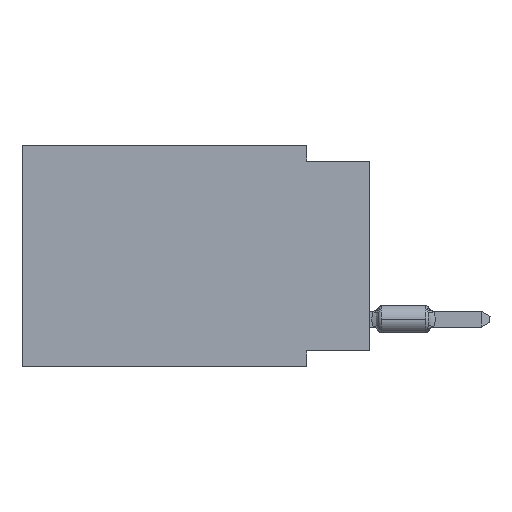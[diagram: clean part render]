
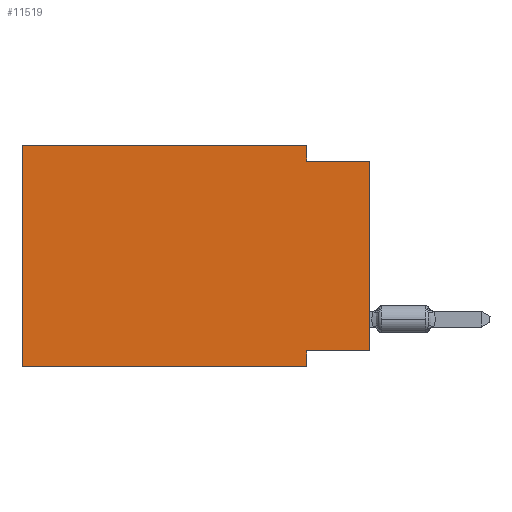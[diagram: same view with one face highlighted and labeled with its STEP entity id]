
A CAD part, left-side view. The second image highlights one B-rep face of the part: STEP entity #11519.
In plain terms, the highlighted planar face has unit normal (-1, 0, 0).
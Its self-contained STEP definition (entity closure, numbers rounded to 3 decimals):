
#225 = EDGE_CURVE ( 'NONE', #2638, #29900, #37555, .T. ) ;
#253 = CARTESIAN_POINT ( 'NONE',  ( 0., 0., -8.255 ) ) ;
#2038 = VECTOR ( 'NONE', #21375, 1000. ) ;
#2461 = CARTESIAN_POINT ( 'NONE',  ( 0., 13.97, -8.89 ) ) ;
#2638 = VERTEX_POINT ( 'NONE', #18817 ) ;
#3577 = DIRECTION ( 'NONE',  ( 1., 0., 0. ) ) ;
#8755 = EDGE_CURVE ( 'NONE', #37932, #35899, #27618, .T. ) ;
#8893 = FACE_OUTER_BOUND ( 'NONE', #53935, .T. ) ;
#9182 = CARTESIAN_POINT ( 'NONE',  ( 0., 2.54, 0. ) ) ;
#10753 = CARTESIAN_POINT ( 'NONE',  ( 0., 2.54, -8.89 ) ) ;
#11464 = VERTEX_POINT ( 'NONE', #9182 ) ;
#11519 = ADVANCED_FACE ( 'NONE', ( #8893 ), #27008, .F. ) ;
#12480 = EDGE_CURVE ( 'NONE', #11464, #40241, #20496, .T. ) ;
#13843 = EDGE_CURVE ( 'NONE', #37932, #29900, #56227, .T. ) ;
#18072 = EDGE_CURVE ( 'NONE', #40241, #25792, #42364, .T. ) ;
#18817 = CARTESIAN_POINT ( 'NONE',  ( 0., 2.54, -8.255 ) ) ;
#18833 = CARTESIAN_POINT ( 'NONE',  ( 0., 2.54, -8.89 ) ) ;
#19452 = CARTESIAN_POINT ( 'NONE',  ( 0., 0., -8.255 ) ) ;
#19778 = CARTESIAN_POINT ( 'NONE',  ( 0., 0., -0.635 ) ) ;
#20298 = VECTOR ( 'NONE', #28694, 1000. ) ;
#20496 = LINE ( 'NONE', #38919, #2038 ) ;
#21157 = VECTOR ( 'NONE', #37764, 1000. ) ;
#21375 = DIRECTION ( 'NONE',  ( 0., 0., -1. ) ) ;
#23720 = AXIS2_PLACEMENT_3D ( 'NONE', #45130, #3577, #57916 ) ;
#25696 = EDGE_CURVE ( 'NONE', #30554, #2638, #42333, .T. ) ;
#25792 = VERTEX_POINT ( 'NONE', #38165 ) ;
#27008 = PLANE ( 'NONE',  #23720 ) ;
#27618 = LINE ( 'NONE', #37426, #53751 ) ;
#28192 = CARTESIAN_POINT ( 'NONE',  ( 0., 13.97, -8.89 ) ) ;
#28514 = LINE ( 'NONE', #51082, #40633 ) ;
#28694 = DIRECTION ( 'NONE',  ( 0., -1., 0. ) ) ;
#29501 = ORIENTED_EDGE ( 'NONE', *, *, #13843, .T. ) ;
#29900 = VERTEX_POINT ( 'NONE', #10753 ) ;
#30554 = VERTEX_POINT ( 'NONE', #253 ) ;
#32705 = CARTESIAN_POINT ( 'NONE',  ( 0., 0., 0. ) ) ;
#33059 = ORIENTED_EDGE ( 'NONE', *, *, #225, .F. ) ;
#33411 = ORIENTED_EDGE ( 'NONE', *, *, #8755, .F. ) ;
#35899 = VERTEX_POINT ( 'NONE', #39149 ) ;
#36910 = VECTOR ( 'NONE', #37587, 1000. ) ;
#37426 = CARTESIAN_POINT ( 'NONE',  ( 0., 13.97, 0. ) ) ;
#37555 = LINE ( 'NONE', #18833, #45721 ) ;
#37587 = DIRECTION ( 'NONE',  ( 0., 1., 0. ) ) ;
#37764 = DIRECTION ( 'NONE',  ( 0., 0., 1. ) ) ;
#37772 = CARTESIAN_POINT ( 'NONE',  ( 0., 2.54, -0.635 ) ) ;
#37932 = VERTEX_POINT ( 'NONE', #28192 ) ;
#38165 = CARTESIAN_POINT ( 'NONE',  ( 0., 0., -0.635 ) ) ;
#38228 = ORIENTED_EDGE ( 'NONE', *, *, #18072, .F. ) ;
#38919 = CARTESIAN_POINT ( 'NONE',  ( 0., 2.54, 0. ) ) ;
#38969 = EDGE_CURVE ( 'NONE', #30554, #25792, #41631, .T. ) ;
#39149 = CARTESIAN_POINT ( 'NONE',  ( 0., 13.97, 0. ) ) ;
#40241 = VERTEX_POINT ( 'NONE', #37772 ) ;
#40633 = VECTOR ( 'NONE', #52232, 1000. ) ;
#41631 = LINE ( 'NONE', #32705, #21157 ) ;
#42333 = LINE ( 'NONE', #19452, #36910 ) ;
#42364 = LINE ( 'NONE', #19778, #20298 ) ;
#45130 = CARTESIAN_POINT ( 'NONE',  ( 0., 13.97, 0. ) ) ;
#45721 = VECTOR ( 'NONE', #55662, 1000. ) ;
#47053 = VECTOR ( 'NONE', #51176, 1000. ) ;
#49844 = ORIENTED_EDGE ( 'NONE', *, *, #38969, .T. ) ;
#51082 = CARTESIAN_POINT ( 'NONE',  ( 0., 13.97, 0. ) ) ;
#51176 = DIRECTION ( 'NONE',  ( 0., -1., 0. ) ) ;
#52232 = DIRECTION ( 'NONE',  ( 0., -1., 0. ) ) ;
#53751 = VECTOR ( 'NONE', #55534, 1000. ) ;
#53935 = EDGE_LOOP ( 'NONE', ( #49844, #38228, #56958, #57719, #33411, #29501, #33059, #57186 ) ) ;
#55406 = EDGE_CURVE ( 'NONE', #35899, #11464, #28514, .T. ) ;
#55534 = DIRECTION ( 'NONE',  ( 0., 0., 1. ) ) ;
#55662 = DIRECTION ( 'NONE',  ( 0., 0., -1. ) ) ;
#56227 = LINE ( 'NONE', #2461, #47053 ) ;
#56958 = ORIENTED_EDGE ( 'NONE', *, *, #12480, .F. ) ;
#57186 = ORIENTED_EDGE ( 'NONE', *, *, #25696, .F. ) ;
#57719 = ORIENTED_EDGE ( 'NONE', *, *, #55406, .F. ) ;
#57916 = DIRECTION ( 'NONE',  ( 0., 0., -1. ) ) ;
